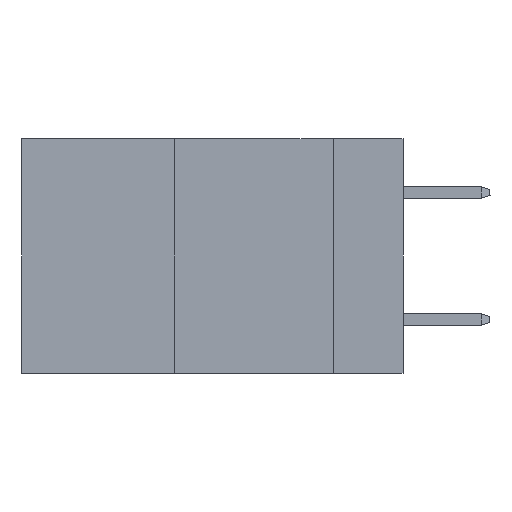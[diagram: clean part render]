
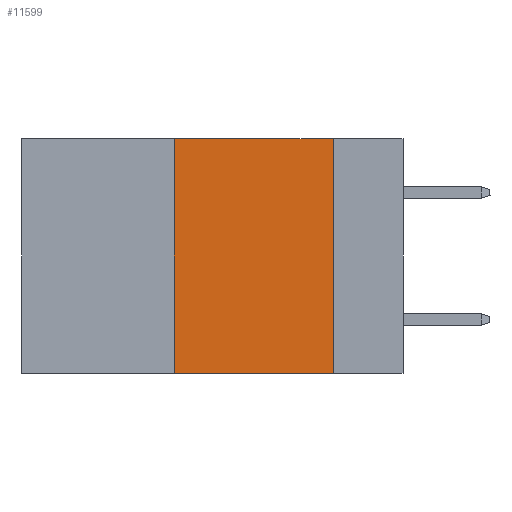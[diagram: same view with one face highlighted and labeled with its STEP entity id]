
A CAD part, left-side view. The second image highlights one B-rep face of the part: STEP entity #11599.
In plain terms, the highlighted planar face has unit normal (-1, 0, 0).
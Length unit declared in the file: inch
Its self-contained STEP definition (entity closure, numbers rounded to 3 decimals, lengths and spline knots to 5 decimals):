
#1291 = ORIENTED_EDGE ( 'NONE', *, *, #13734, .F. ) ;
#2618 = CARTESIAN_POINT ( 'NONE',  ( 0., 0.36, 0. ) ) ;
#3800 = VECTOR ( 'NONE', #4673, 39.37008 ) ;
#3850 = CARTESIAN_POINT ( 'NONE',  ( 0., 0.6, 0. ) ) ;
#4673 = DIRECTION ( 'NONE',  ( 0., -1., 0. ) ) ;
#5134 = ORIENTED_EDGE ( 'NONE', *, *, #7141, .T. ) ;
#5403 = PLANE ( 'NONE',  #8418 ) ;
#6312 = VERTEX_POINT ( 'NONE', #15303 ) ;
#6334 = CARTESIAN_POINT ( 'NONE',  ( 0., 0.36, -0.37 ) ) ;
#7141 = EDGE_CURVE ( 'NONE', #8039, #16084, #7160, .T. ) ;
#7160 = LINE ( 'NONE', #8766, #3800 ) ;
#7832 = DIRECTION ( 'NONE',  ( 0., 0., -1. ) ) ;
#8039 = VERTEX_POINT ( 'NONE', #6334 ) ;
#8270 = VECTOR ( 'NONE', #7832, 39.37008 ) ;
#8348 = CARTESIAN_POINT ( 'NONE',  ( 0., 0.11, -0.37 ) ) ;
#8418 = AXIS2_PLACEMENT_3D ( 'NONE', #3850, #12825, #11721 ) ;
#8504 = VECTOR ( 'NONE', #14151, 39.37008 ) ;
#8593 = EDGE_CURVE ( 'NONE', #14191, #16084, #14330, .T. ) ;
#8766 = CARTESIAN_POINT ( 'NONE',  ( 0., 0.6, -0.37 ) ) ;
#10233 = LINE ( 'NONE', #2618, #8504 ) ;
#10279 = CARTESIAN_POINT ( 'NONE',  ( 0., 0.11, 0. ) ) ;
#10729 = LINE ( 'NONE', #15767, #15285 ) ;
#11599 = ADVANCED_FACE ( 'NONE', ( #14187 ), #5403, .F. ) ;
#11721 = DIRECTION ( 'NONE',  ( 0., 0., -1. ) ) ;
#12135 = EDGE_CURVE ( 'NONE', #6312, #14191, #10729, .T. ) ;
#12381 = EDGE_LOOP ( 'NONE', ( #15078, #14771, #1291, #5134 ) ) ;
#12825 = DIRECTION ( 'NONE',  ( 1., 0., 0. ) ) ;
#13734 = EDGE_CURVE ( 'NONE', #8039, #6312, #10233, .T. ) ;
#14151 = DIRECTION ( 'NONE',  ( 0., 0., 1. ) ) ;
#14187 = FACE_OUTER_BOUND ( 'NONE', #12381, .T. ) ;
#14191 = VERTEX_POINT ( 'NONE', #10279 ) ;
#14330 = LINE ( 'NONE', #16827, #8270 ) ;
#14771 = ORIENTED_EDGE ( 'NONE', *, *, #12135, .F. ) ;
#15078 = ORIENTED_EDGE ( 'NONE', *, *, #8593, .F. ) ;
#15285 = VECTOR ( 'NONE', #15934, 39.37008 ) ;
#15303 = CARTESIAN_POINT ( 'NONE',  ( 0., 0.36, 0. ) ) ;
#15767 = CARTESIAN_POINT ( 'NONE',  ( 0., 0.6, 0. ) ) ;
#15934 = DIRECTION ( 'NONE',  ( 0., -1., 0. ) ) ;
#16084 = VERTEX_POINT ( 'NONE', #8348 ) ;
#16827 = CARTESIAN_POINT ( 'NONE',  ( 0., 0.11, 0. ) ) ;
